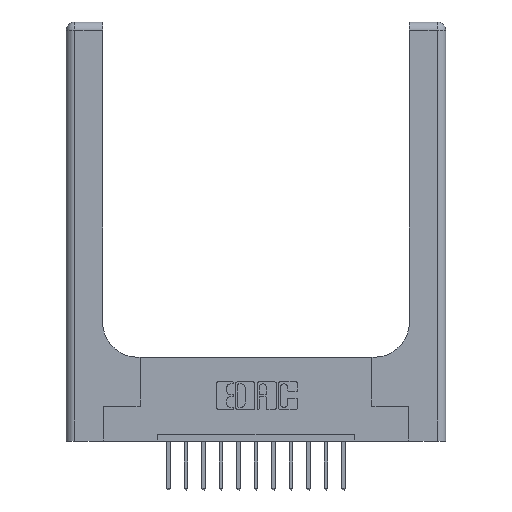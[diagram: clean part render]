
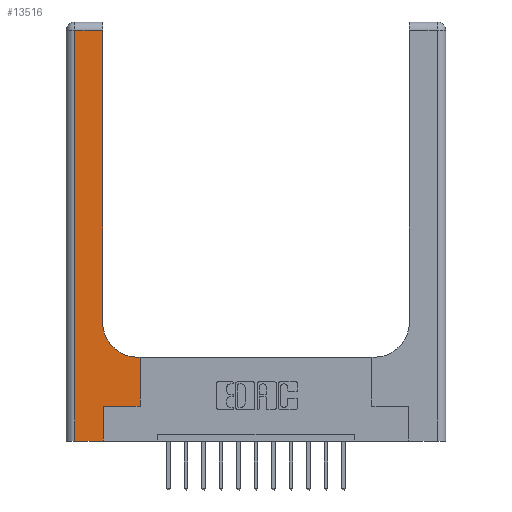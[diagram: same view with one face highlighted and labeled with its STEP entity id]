
A CAD part, top view. The second image highlights one B-rep face of the part: STEP entity #13516.
In plain terms, the highlighted planar face has unit normal (0, 0, 1).
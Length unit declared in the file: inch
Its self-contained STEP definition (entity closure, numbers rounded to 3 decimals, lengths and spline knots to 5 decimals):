
#217 = CARTESIAN_POINT ( 'NONE',  ( 0.51, 0.6, 0.37 ) ) ;
#274 = VERTEX_POINT ( 'NONE', #13814 ) ;
#285 = VECTOR ( 'NONE', #15658, 39.37008 ) ;
#525 = EDGE_CURVE ( 'NONE', #9768, #14979, #13918, .T. ) ;
#658 = CARTESIAN_POINT ( 'NONE',  ( 0.265, 0., 0.37 ) ) ;
#746 = ORIENTED_EDGE ( 'NONE', *, *, #12621, .T. ) ;
#952 = AXIS2_PLACEMENT_3D ( 'NONE', #15177, #12854, #14043 ) ;
#1189 = CARTESIAN_POINT ( 'NONE',  ( 0., 3., 0.37 ) ) ;
#1231 = FACE_OUTER_BOUND ( 'NONE', #14438, .T. ) ;
#1712 = DIRECTION ( 'NONE',  ( -1., 0., 0. ) ) ;
#1977 = CARTESIAN_POINT ( 'NONE',  ( 0.265, 0.25, 0.37 ) ) ;
#2200 = CARTESIAN_POINT ( 'NONE',  ( 0.06, 3., 0.37 ) ) ;
#2207 = VECTOR ( 'NONE', #11192, 39.37008 ) ;
#3046 = VERTEX_POINT ( 'NONE', #10563 ) ;
#3157 = LINE ( 'NONE', #2200, #13694 ) ;
#3361 = LINE ( 'NONE', #15901, #7403 ) ;
#3592 = DIRECTION ( 'NONE',  ( 0., 1., 0. ) ) ;
#3848 = ORIENTED_EDGE ( 'NONE', *, *, #11257, .T. ) ;
#3951 = ORIENTED_EDGE ( 'NONE', *, *, #15427, .T. ) ;
#4450 = DIRECTION ( 'NONE',  ( 1., 0., 0. ) ) ;
#4708 = ORIENTED_EDGE ( 'NONE', *, *, #5331, .T. ) ;
#4927 = LINE ( 'NONE', #9979, #2207 ) ;
#5331 = EDGE_CURVE ( 'NONE', #11900, #8836, #7765, .T. ) ;
#5477 = VECTOR ( 'NONE', #10177, 39.37008 ) ;
#6198 = DIRECTION ( 'NONE',  ( 0., 0., -1. ) ) ;
#6538 = ORIENTED_EDGE ( 'NONE', *, *, #13464, .T. ) ;
#6627 = DIRECTION ( 'NONE',  ( 0., 1., 0. ) ) ;
#6904 = LINE ( 'NONE', #10720, #285 ) ;
#7403 = VECTOR ( 'NONE', #3592, 39.37008 ) ;
#7605 = VERTEX_POINT ( 'NONE', #217 ) ;
#7765 = LINE ( 'NONE', #14041, #9346 ) ;
#8137 = ORIENTED_EDGE ( 'NONE', *, *, #11610, .T. ) ;
#8401 = ORIENTED_EDGE ( 'NONE', *, *, #525, .T. ) ;
#8455 = DIRECTION ( 'NONE',  ( 0., -1., 0. ) ) ;
#8828 = PLANE ( 'NONE',  #11536 ) ;
#8829 = CARTESIAN_POINT ( 'NONE',  ( 0.528, 0.25, 0.37 ) ) ;
#8836 = VERTEX_POINT ( 'NONE', #11896 ) ;
#8876 = VERTEX_POINT ( 'NONE', #9303 ) ;
#9303 = CARTESIAN_POINT ( 'NONE',  ( 0.26, 0.85, 0.37 ) ) ;
#9346 = VECTOR ( 'NONE', #6627, 39.37008 ) ;
#9390 = VECTOR ( 'NONE', #4450, 39.37008 ) ;
#9768 = VERTEX_POINT ( 'NONE', #14307 ) ;
#9979 = CARTESIAN_POINT ( 'NONE',  ( 0.26, 0.6, 0.37 ) ) ;
#10177 = DIRECTION ( 'NONE',  ( 0., 1., 0. ) ) ;
#10563 = CARTESIAN_POINT ( 'NONE',  ( 0.06, 2.94, 0.37 ) ) ;
#10647 = CARTESIAN_POINT ( 'NONE',  ( 0., 2.94, 0.37 ) ) ;
#10720 = CARTESIAN_POINT ( 'NONE',  ( 0.265, 0.25, 0.37 ) ) ;
#10743 = EDGE_CURVE ( 'NONE', #14979, #13418, #15065, .T. ) ;
#10765 = CIRCLE ( 'NONE', #952, 0.25 ) ;
#11192 = DIRECTION ( 'NONE',  ( -1., 0., 0. ) ) ;
#11257 = EDGE_CURVE ( 'NONE', #3046, #9768, #3157, .T. ) ;
#11366 = DIRECTION ( 'NONE',  ( -1., 0., 0. ) ) ;
#11402 = CARTESIAN_POINT ( 'NONE',  ( 0.265, 0., 0.37 ) ) ;
#11536 = AXIS2_PLACEMENT_3D ( 'NONE', #1189, #6198, #11366 ) ;
#11610 = EDGE_CURVE ( 'NONE', #274, #3046, #13316, .T. ) ;
#11896 = CARTESIAN_POINT ( 'NONE',  ( 0.528, 0.6, 0.37 ) ) ;
#11900 = VERTEX_POINT ( 'NONE', #8829 ) ;
#12621 = EDGE_CURVE ( 'NONE', #13418, #11900, #6904, .T. ) ;
#12817 = ORIENTED_EDGE ( 'NONE', *, *, #15137, .T. ) ;
#12854 = DIRECTION ( 'NONE',  ( 0., 0., -1. ) ) ;
#13279 = CARTESIAN_POINT ( 'NONE',  ( 0., 0., 0.37 ) ) ;
#13304 = VECTOR ( 'NONE', #1712, 39.37008 ) ;
#13316 = LINE ( 'NONE', #10647, #13304 ) ;
#13418 = VERTEX_POINT ( 'NONE', #1977 ) ;
#13464 = EDGE_CURVE ( 'NONE', #8836, #7605, #4927, .T. ) ;
#13516 = ADVANCED_FACE ( 'NONE', ( #1231 ), #8828, .F. ) ;
#13694 = VECTOR ( 'NONE', #8455, 39.37008 ) ;
#13814 = CARTESIAN_POINT ( 'NONE',  ( 0.26, 2.94, 0.37 ) ) ;
#13918 = LINE ( 'NONE', #13279, #9390 ) ;
#14041 = CARTESIAN_POINT ( 'NONE',  ( 0.528, 0.25, 0.37 ) ) ;
#14043 = DIRECTION ( 'NONE',  ( 1., 0., 0. ) ) ;
#14307 = CARTESIAN_POINT ( 'NONE',  ( 0.06, 0., 0.37 ) ) ;
#14438 = EDGE_LOOP ( 'NONE', ( #12817, #8137, #3848, #8401, #14515, #746, #4708, #6538, #3951 ) ) ;
#14515 = ORIENTED_EDGE ( 'NONE', *, *, #10743, .T. ) ;
#14979 = VERTEX_POINT ( 'NONE', #658 ) ;
#15065 = LINE ( 'NONE', #11402, #5477 ) ;
#15137 = EDGE_CURVE ( 'NONE', #8876, #274, #3361, .T. ) ;
#15177 = CARTESIAN_POINT ( 'NONE',  ( 0.51, 0.85, 0.37 ) ) ;
#15427 = EDGE_CURVE ( 'NONE', #7605, #8876, #10765, .T. ) ;
#15658 = DIRECTION ( 'NONE',  ( 1., 0., 0. ) ) ;
#15901 = CARTESIAN_POINT ( 'NONE',  ( 0.26, 3., 0.37 ) ) ;
